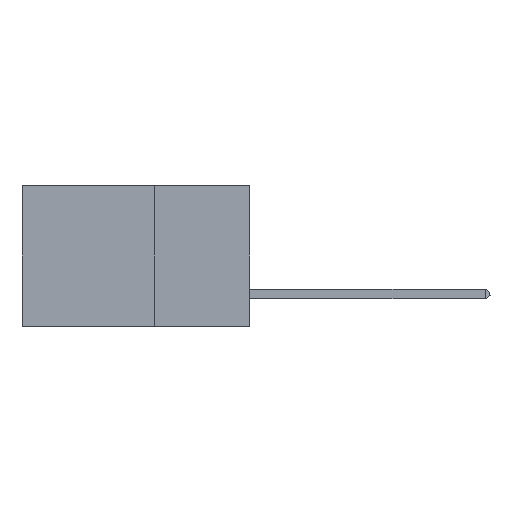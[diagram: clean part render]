
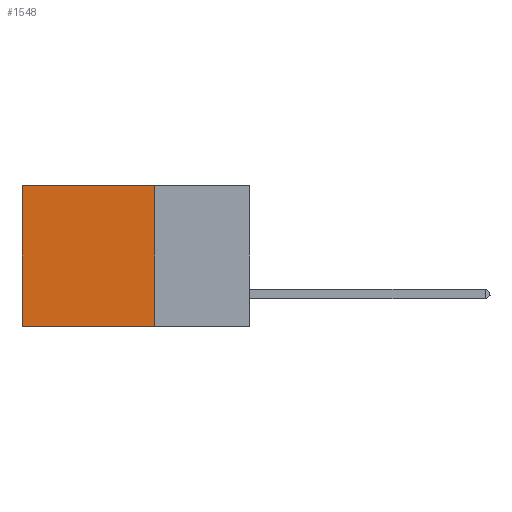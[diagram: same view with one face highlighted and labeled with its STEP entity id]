
A CAD part, left-side view. The second image highlights one B-rep face of the part: STEP entity #1548.
In plain terms, the highlighted planar face has unit normal (-1, 0, 0).
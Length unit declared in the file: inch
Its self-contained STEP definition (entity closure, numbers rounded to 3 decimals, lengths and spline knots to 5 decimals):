
#1056 = DIRECTION ( 'NONE',  ( 0., 1., 0. ) ) ;
#1318 = AXIS2_PLACEMENT_3D ( 'NONE', #46349, #12652, #39356 ) ;
#1332 = VECTOR ( 'NONE', #1056, 39.37008 ) ;
#1548 = ADVANCED_FACE ( 'NONE', ( #5079 ), #46520, .F. ) ;
#3662 = CARTESIAN_POINT ( 'NONE',  ( 0.2875, 0.6, 0. ) ) ;
#5079 = FACE_OUTER_BOUND ( 'NONE', #20193, .T. ) ;
#6262 = CARTESIAN_POINT ( 'NONE',  ( 0.2875, 0.6, -0.37 ) ) ;
#7738 = DIRECTION ( 'NONE',  ( 0., 1., 0. ) ) ;
#10986 = VERTEX_POINT ( 'NONE', #3662 ) ;
#11855 = ORIENTED_EDGE ( 'NONE', *, *, #39804, .T. ) ;
#12652 = DIRECTION ( 'NONE',  ( 1., 0., 0. ) ) ;
#12924 = LINE ( 'NONE', #35042, #36841 ) ;
#12957 = VERTEX_POINT ( 'NONE', #6262 ) ;
#14604 = EDGE_CURVE ( 'NONE', #25947, #12957, #24656, .T. ) ;
#15037 = CARTESIAN_POINT ( 'NONE',  ( 0.2875, 0.25, -0.37 ) ) ;
#15960 = DIRECTION ( 'NONE',  ( 0., 0., -1. ) ) ;
#16658 = ORIENTED_EDGE ( 'NONE', *, *, #48211, .T. ) ;
#17149 = VECTOR ( 'NONE', #15960, 39.37008 ) ;
#17432 = EDGE_CURVE ( 'NONE', #26450, #25947, #46877, .T. ) ;
#20193 = EDGE_LOOP ( 'NONE', ( #16658, #29999, #43998, #11855 ) ) ;
#24656 = LINE ( 'NONE', #42307, #1332 ) ;
#25947 = VERTEX_POINT ( 'NONE', #15037 ) ;
#26450 = VERTEX_POINT ( 'NONE', #41985 ) ;
#27007 = CARTESIAN_POINT ( 'NONE',  ( 0.2875, 0.25, 0. ) ) ;
#29999 = ORIENTED_EDGE ( 'NONE', *, *, #14604, .F. ) ;
#32547 = DIRECTION ( 'NONE',  ( 0., 0., -1. ) ) ;
#35042 = CARTESIAN_POINT ( 'NONE',  ( 0.2875, 0.6, 0. ) ) ;
#36394 = VECTOR ( 'NONE', #7738, 39.37008 ) ;
#36841 = VECTOR ( 'NONE', #32547, 39.37008 ) ;
#39356 = DIRECTION ( 'NONE',  ( 0., 0., -1. ) ) ;
#39804 = EDGE_CURVE ( 'NONE', #26450, #10986, #46315, .T. ) ;
#41035 = CARTESIAN_POINT ( 'NONE',  ( 0.2875, 0.25, 0. ) ) ;
#41985 = CARTESIAN_POINT ( 'NONE',  ( 0.2875, 0.25, 0. ) ) ;
#42307 = CARTESIAN_POINT ( 'NONE',  ( 0.2875, 0.25, -0.37 ) ) ;
#43998 = ORIENTED_EDGE ( 'NONE', *, *, #17432, .F. ) ;
#46315 = LINE ( 'NONE', #41035, #36394 ) ;
#46349 = CARTESIAN_POINT ( 'NONE',  ( 0.2875, 0.25, 0. ) ) ;
#46520 = PLANE ( 'NONE',  #1318 ) ;
#46877 = LINE ( 'NONE', #27007, #17149 ) ;
#48211 = EDGE_CURVE ( 'NONE', #10986, #12957, #12924, .T. ) ;
